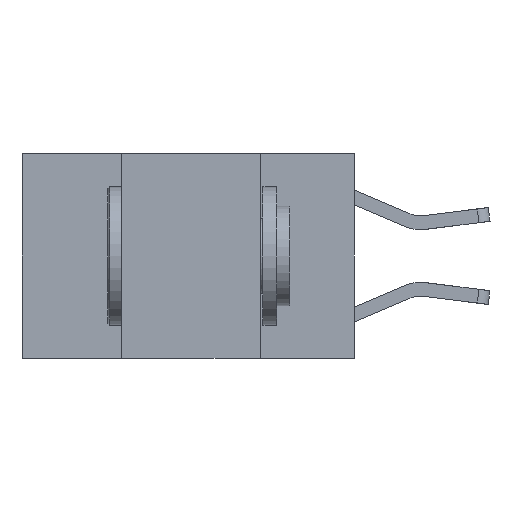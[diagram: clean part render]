
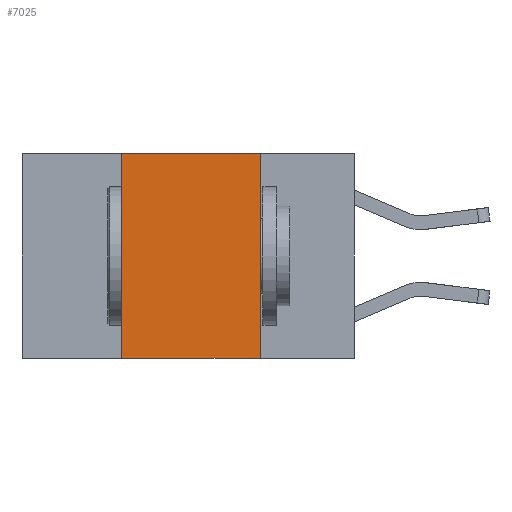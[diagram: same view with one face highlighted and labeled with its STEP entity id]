
A CAD part, left-side view. The second image highlights one B-rep face of the part: STEP entity #7025.
In plain terms, the highlighted planar face has unit normal (-1, 0, 0).
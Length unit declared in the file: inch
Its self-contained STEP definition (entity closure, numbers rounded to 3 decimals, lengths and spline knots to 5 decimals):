
#98 = VECTOR ( 'NONE', #7681, 39.37008 ) ;
#268 = LINE ( 'NONE', #6201, #5875 ) ;
#598 = CARTESIAN_POINT ( 'NONE',  ( 0., 0.6, 0. ) ) ;
#600 = LINE ( 'NONE', #6847, #9586 ) ;
#987 = EDGE_CURVE ( 'NONE', #8994, #4449, #3092, .T. ) ;
#1319 = ORIENTED_EDGE ( 'NONE', *, *, #7865, .T. ) ;
#1534 = FACE_OUTER_BOUND ( 'NONE', #5914, .T. ) ;
#1802 = EDGE_CURVE ( 'NONE', #4449, #7922, #3463, .T. ) ;
#3092 = LINE ( 'NONE', #6137, #98 ) ;
#3289 = DIRECTION ( 'NONE',  ( 0., 0., -1. ) ) ;
#3449 = ORIENTED_EDGE ( 'NONE', *, *, #1802, .F. ) ;
#3463 = LINE ( 'NONE', #598, #4526 ) ;
#3464 = AXIS2_PLACEMENT_3D ( 'NONE', #4443, #8355, #4546 ) ;
#4443 = CARTESIAN_POINT ( 'NONE',  ( 0., 0.6, 0. ) ) ;
#4449 = VERTEX_POINT ( 'NONE', #9859 ) ;
#4526 = VECTOR ( 'NONE', #8834, 39.37008 ) ;
#4546 = DIRECTION ( 'NONE',  ( 0., 0., -1. ) ) ;
#5228 = DIRECTION ( 'NONE',  ( 0., -1., 0. ) ) ;
#5481 = ORIENTED_EDGE ( 'NONE', *, *, #987, .F. ) ;
#5828 = EDGE_CURVE ( 'NONE', #7922, #5833, #268, .T. ) ;
#5833 = VERTEX_POINT ( 'NONE', #8548 ) ;
#5875 = VECTOR ( 'NONE', #3289, 39.37008 ) ;
#5914 = EDGE_LOOP ( 'NONE', ( #6776, #3449, #5481, #1319 ) ) ;
#6027 = CARTESIAN_POINT ( 'NONE',  ( 0., 0.17, 0. ) ) ;
#6055 = PLANE ( 'NONE',  #3464 ) ;
#6137 = CARTESIAN_POINT ( 'NONE',  ( 0., 0.42, 0. ) ) ;
#6159 = CARTESIAN_POINT ( 'NONE',  ( 0., 0.42, -0.37 ) ) ;
#6201 = CARTESIAN_POINT ( 'NONE',  ( 0., 0.17, 0. ) ) ;
#6776 = ORIENTED_EDGE ( 'NONE', *, *, #5828, .F. ) ;
#6847 = CARTESIAN_POINT ( 'NONE',  ( 0., 0.6, -0.37 ) ) ;
#7025 = ADVANCED_FACE ( 'NONE', ( #1534 ), #6055, .F. ) ;
#7681 = DIRECTION ( 'NONE',  ( 0., 0., 1. ) ) ;
#7865 = EDGE_CURVE ( 'NONE', #8994, #5833, #600, .T. ) ;
#7922 = VERTEX_POINT ( 'NONE', #6027 ) ;
#8355 = DIRECTION ( 'NONE',  ( 1., 0., 0. ) ) ;
#8548 = CARTESIAN_POINT ( 'NONE',  ( 0., 0.17, -0.37 ) ) ;
#8834 = DIRECTION ( 'NONE',  ( 0., -1., 0. ) ) ;
#8994 = VERTEX_POINT ( 'NONE', #6159 ) ;
#9586 = VECTOR ( 'NONE', #5228, 39.37008 ) ;
#9859 = CARTESIAN_POINT ( 'NONE',  ( 0., 0.42, 0. ) ) ;
